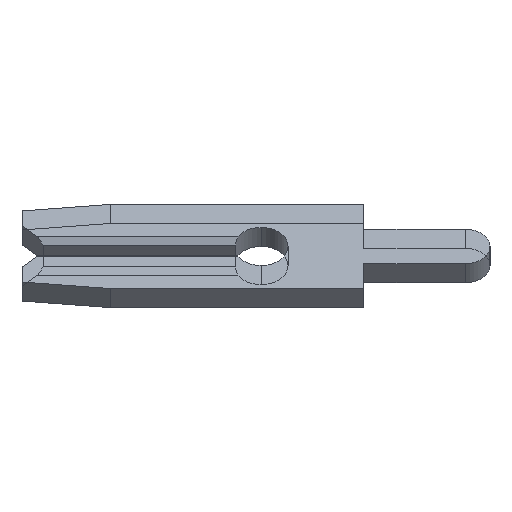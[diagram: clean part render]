
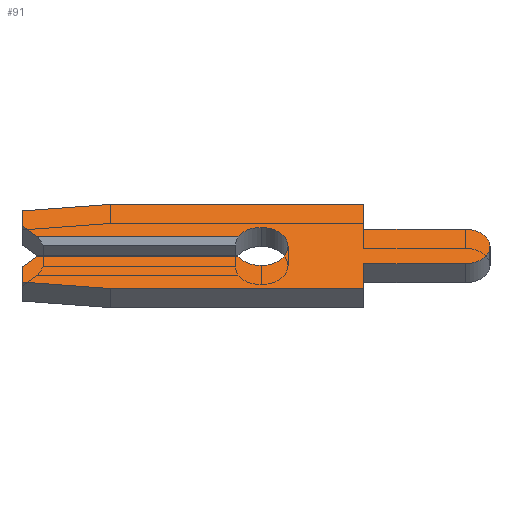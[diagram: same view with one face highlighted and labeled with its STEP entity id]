
A CAD part, left-side view. The second image highlights one B-rep face of the part: STEP entity #91.
In plain terms, the highlighted face is planar.
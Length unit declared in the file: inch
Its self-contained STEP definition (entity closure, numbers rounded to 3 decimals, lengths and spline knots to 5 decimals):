
#60 = CARTESIAN_POINT ( 'NONE',  ( -0.013, -0.099, -0.0235 ) ) ;
#91 = ADVANCED_FACE ( 'NONE', ( #1118 ), #2177, .F. ) ;
#99 = VERTEX_POINT ( 'NONE', #2155 ) ;
#103 = CARTESIAN_POINT ( 'NONE',  ( -0.013, 0.146, 0.0575 ) ) ;
#112 = CARTESIAN_POINT ( 'NONE',  ( -0.013, -0.099, 0.0235 ) ) ;
#117 = ORIENTED_EDGE ( 'NONE', *, *, #1726, .F. ) ;
#126 = VECTOR ( 'NONE', #705, 39.37008 ) ;
#244 = DIRECTION ( 'NONE',  ( -1., 0., 0. ) ) ;
#257 = CARTESIAN_POINT ( 'NONE',  ( -0.013, -0.099, -0.0575 ) ) ;
#270 = DIRECTION ( 'NONE',  ( 0., 0., -1. ) ) ;
#275 = ORIENTED_EDGE ( 'NONE', *, *, #1500, .F. ) ;
#277 = AXIS2_PLACEMENT_3D ( 'NONE', #1035, #1986, #2383 ) ;
#281 = VECTOR ( 'NONE', #2436, 39.37008 ) ;
#286 = VERTEX_POINT ( 'NONE', #1209 ) ;
#304 = CARTESIAN_POINT ( 'NONE',  ( -0.013, 0.231, 0.013 ) ) ;
#312 = VECTOR ( 'NONE', #2192, 39.37008 ) ;
#326 = EDGE_CURVE ( 'NONE', #1054, #760, #437, .T. ) ;
#342 = CIRCLE ( 'NONE', #898, 0.026 ) ;
#346 = CARTESIAN_POINT ( 'NONE',  ( -0.013, 0.216, -0.013 ) ) ;
#365 = LINE ( 'NONE', #1423, #1290 ) ;
#419 = LINE ( 'NONE', #2057, #1211 ) ;
#423 = DIRECTION ( 'NONE',  ( 0., 0., -1. ) ) ;
#432 = ORIENTED_EDGE ( 'NONE', *, *, #2236, .F. ) ;
#434 = VECTOR ( 'NONE', #1541, 39.37008 ) ;
#437 = LINE ( 'NONE', #1969, #2438 ) ;
#481 = EDGE_CURVE ( 'NONE', #649, #2296, #1342, .T. ) ;
#502 = LINE ( 'NONE', #1809, #1107 ) ;
#508 = CIRCLE ( 'NONE', #2370, 0.0235 ) ;
#511 = DIRECTION ( 'NONE',  ( -1., 0., 0. ) ) ;
#542 = LINE ( 'NONE', #908, #434 ) ;
#558 = ORIENTED_EDGE ( 'NONE', *, *, #858, .F. ) ;
#614 = DIRECTION ( 'NONE',  ( 0., -1., 0. ) ) ;
#634 = ORIENTED_EDGE ( 'NONE', *, *, #1562, .F. ) ;
#649 = VERTEX_POINT ( 'NONE', #60 ) ;
#651 = CARTESIAN_POINT ( 'NONE',  ( -0.013, 0., 0. ) ) ;
#661 = VECTOR ( 'NONE', #2313, 39.37008 ) ;
#692 = VERTEX_POINT ( 'NONE', #1614 ) ;
#705 = DIRECTION ( 'NONE',  ( 0., -1., 0. ) ) ;
#708 = CARTESIAN_POINT ( 'NONE',  ( -0.013, 0.02252, -0.013 ) ) ;
#726 = EDGE_CURVE ( 'NONE', #1320, #2247, #1497, .T. ) ;
#737 = CARTESIAN_POINT ( 'NONE',  ( -0.013, 0.231, -0.028 ) ) ;
#760 = VERTEX_POINT ( 'NONE', #2228 ) ;
#766 = CARTESIAN_POINT ( 'NONE',  ( -0.013, 0.2105, -0.0075 ) ) ;
#819 = LINE ( 'NONE', #766, #853 ) ;
#828 = EDGE_CURVE ( 'NONE', #692, #2247, #342, .T. ) ;
#845 = VERTEX_POINT ( 'NONE', #103 ) ;
#853 = VECTOR ( 'NONE', #1145, 39.37008 ) ;
#858 = EDGE_CURVE ( 'NONE', #1320, #1738, #1746, .T. ) ;
#898 = AXIS2_PLACEMENT_3D ( 'NONE', #2047, #511, #1663 ) ;
#908 = CARTESIAN_POINT ( 'NONE',  ( -0.013, 0., -0.013 ) ) ;
#970 = CARTESIAN_POINT ( 'NONE',  ( -0.013, 0.146, -0.0575 ) ) ;
#1035 = CARTESIAN_POINT ( 'NONE',  ( -0.013, 0., 0. ) ) ;
#1050 = CARTESIAN_POINT ( 'NONE',  ( -0.013, -0.1975, 0. ) ) ;
#1054 = VERTEX_POINT ( 'NONE', #112 ) ;
#1061 = VECTOR ( 'NONE', #1539, 39.37008 ) ;
#1098 = CARTESIAN_POINT ( 'NONE',  ( -0.013, 0.231, -0.04857 ) ) ;
#1106 = VECTOR ( 'NONE', #1156, 39.37008 ) ;
#1107 = VECTOR ( 'NONE', #1991, 39.37008 ) ;
#1118 = FACE_OUTER_BOUND ( 'NONE', #1835, .T. ) ;
#1127 = EDGE_CURVE ( 'NONE', #845, #99, #419, .T. ) ;
#1145 = DIRECTION ( 'NONE',  ( 0., -0.707, 0.707 ) ) ;
#1156 = DIRECTION ( 'NONE',  ( 0., 1., 0. ) ) ;
#1158 = ORIENTED_EDGE ( 'NONE', *, *, #1813, .F. ) ;
#1181 = DIRECTION ( 'NONE',  ( 0., 0., -1. ) ) ;
#1185 = CARTESIAN_POINT ( 'NONE',  ( -0.013, 0.231, 0.028 ) ) ;
#1202 = ORIENTED_EDGE ( 'NONE', *, *, #326, .F. ) ;
#1205 = VECTOR ( 'NONE', #2275, 39.37008 ) ;
#1206 = ORIENTED_EDGE ( 'NONE', *, *, #2458, .F. ) ;
#1209 = CARTESIAN_POINT ( 'NONE',  ( -0.013, 0., -0.026 ) ) ;
#1211 = VECTOR ( 'NONE', #1296, 39.37008 ) ;
#1233 = VERTEX_POINT ( 'NONE', #346 ) ;
#1245 = CARTESIAN_POINT ( 'NONE',  ( -0.013, 0.231, -0.028 ) ) ;
#1257 = CARTESIAN_POINT ( 'NONE',  ( -0.013, 0.231, 0.04857 ) ) ;
#1260 = ORIENTED_EDGE ( 'NONE', *, *, #828, .F. ) ;
#1290 = VECTOR ( 'NONE', #270, 39.37008 ) ;
#1296 = DIRECTION ( 'NONE',  ( 0., -1., 0. ) ) ;
#1320 = VERTEX_POINT ( 'NONE', #1929 ) ;
#1335 = EDGE_CURVE ( 'NONE', #2305, #2015, #1534, .T. ) ;
#1342 = LINE ( 'NONE', #257, #312 ) ;
#1367 = VERTEX_POINT ( 'NONE', #2285 ) ;
#1374 = CARTESIAN_POINT ( 'NONE',  ( -0.013, -0.099, -0.0235 ) ) ;
#1384 = DIRECTION ( 'NONE',  ( 0., 0., 1. ) ) ;
#1423 = CARTESIAN_POINT ( 'NONE',  ( -0.013, -0.099, 0.0575 ) ) ;
#1428 = EDGE_CURVE ( 'NONE', #2015, #1233, #819, .T. ) ;
#1436 = ORIENTED_EDGE ( 'NONE', *, *, #1127, .F. ) ;
#1442 = ORIENTED_EDGE ( 'NONE', *, *, #726, .T. ) ;
#1483 = CARTESIAN_POINT ( 'NONE',  ( -0.013, 0.2105, 0.0075 ) ) ;
#1497 = LINE ( 'NONE', #304, #126 ) ;
#1500 = EDGE_CURVE ( 'NONE', #2301, #286, #2125, .T. ) ;
#1528 = CIRCLE ( 'NONE', #2007, 0.026 ) ;
#1534 = LINE ( 'NONE', #737, #1205 ) ;
#1539 = DIRECTION ( 'NONE',  ( 0., 0., 1. ) ) ;
#1541 = DIRECTION ( 'NONE',  ( 0., -1., 0. ) ) ;
#1548 = CARTESIAN_POINT ( 'NONE',  ( -0.013, 0., 0. ) ) ;
#1562 = EDGE_CURVE ( 'NONE', #1738, #2212, #2016, .T. ) ;
#1570 = VECTOR ( 'NONE', #2343, 39.37008 ) ;
#1578 = CARTESIAN_POINT ( 'NONE',  ( -0.013, 0.146, -0.0575 ) ) ;
#1603 = DIRECTION ( 'NONE',  ( 1., 0., 0. ) ) ;
#1611 = VERTEX_POINT ( 'NONE', #1578 ) ;
#1614 = CARTESIAN_POINT ( 'NONE',  ( -0.013, 0., 0.026 ) ) ;
#1619 = ORIENTED_EDGE ( 'NONE', *, *, #1794, .F. ) ;
#1663 = DIRECTION ( 'NONE',  ( 0., 0., -1. ) ) ;
#1689 = LINE ( 'NONE', #2148, #1570 ) ;
#1692 = EDGE_CURVE ( 'NONE', #2212, #845, #1689, .T. ) ;
#1722 = AXIS2_PLACEMENT_3D ( 'NONE', #1548, #2128, #1181 ) ;
#1726 = EDGE_CURVE ( 'NONE', #2296, #1611, #2412, .T. ) ;
#1738 = VERTEX_POINT ( 'NONE', #1792 ) ;
#1746 = LINE ( 'NONE', #1483, #281 ) ;
#1792 = CARTESIAN_POINT ( 'NONE',  ( -0.013, 0.231, 0.028 ) ) ;
#1794 = EDGE_CURVE ( 'NONE', #286, #692, #1528, .T. ) ;
#1809 = CARTESIAN_POINT ( 'NONE',  ( -0.013, 0.231, -0.04857 ) ) ;
#1813 = EDGE_CURVE ( 'NONE', #760, #1367, #508, .T. ) ;
#1835 = EDGE_LOOP ( 'NONE', ( #1442, #1260, #1619, #275, #1206, #2242, #1996, #2179, #117, #2214, #2091, #1158, #1202, #432, #1436, #1898, #634, #558 ) ) ;
#1845 = LINE ( 'NONE', #1374, #1106 ) ;
#1869 = EDGE_CURVE ( 'NONE', #1611, #2305, #502, .T. ) ;
#1898 = ORIENTED_EDGE ( 'NONE', *, *, #1692, .F. ) ;
#1929 = CARTESIAN_POINT ( 'NONE',  ( -0.013, 0.216, 0.013 ) ) ;
#1969 = CARTESIAN_POINT ( 'NONE',  ( -0.013, -0.099, 0.0235 ) ) ;
#1986 = DIRECTION ( 'NONE',  ( 1., 0., 0. ) ) ;
#1991 = DIRECTION ( 'NONE',  ( 0., 0.995, 0.105 ) ) ;
#1996 = ORIENTED_EDGE ( 'NONE', *, *, #1335, .F. ) ;
#2007 = AXIS2_PLACEMENT_3D ( 'NONE', #651, #244, #423 ) ;
#2015 = VERTEX_POINT ( 'NONE', #1245 ) ;
#2016 = LINE ( 'NONE', #1185, #1061 ) ;
#2047 = CARTESIAN_POINT ( 'NONE',  ( -0.013, 0., 0. ) ) ;
#2057 = CARTESIAN_POINT ( 'NONE',  ( -0.013, 0.146, 0.0575 ) ) ;
#2091 = ORIENTED_EDGE ( 'NONE', *, *, #2445, .F. ) ;
#2125 = CIRCLE ( 'NONE', #1722, 0.026 ) ;
#2128 = DIRECTION ( 'NONE',  ( -1., 0., 0. ) ) ;
#2148 = CARTESIAN_POINT ( 'NONE',  ( -0.013, 0.231, 0.04857 ) ) ;
#2155 = CARTESIAN_POINT ( 'NONE',  ( -0.013, -0.099, 0.0575 ) ) ;
#2177 = PLANE ( 'NONE',  #277 ) ;
#2179 = ORIENTED_EDGE ( 'NONE', *, *, #1869, .F. ) ;
#2192 = DIRECTION ( 'NONE',  ( 0., 0., -1. ) ) ;
#2212 = VERTEX_POINT ( 'NONE', #1257 ) ;
#2214 = ORIENTED_EDGE ( 'NONE', *, *, #481, .F. ) ;
#2228 = CARTESIAN_POINT ( 'NONE',  ( -0.013, -0.1975, 0.0235 ) ) ;
#2236 = EDGE_CURVE ( 'NONE', #99, #1054, #365, .T. ) ;
#2242 = ORIENTED_EDGE ( 'NONE', *, *, #1428, .F. ) ;
#2247 = VERTEX_POINT ( 'NONE', #2433 ) ;
#2275 = DIRECTION ( 'NONE',  ( 0., 0., 1. ) ) ;
#2285 = CARTESIAN_POINT ( 'NONE',  ( -0.013, -0.1975, -0.0235 ) ) ;
#2296 = VERTEX_POINT ( 'NONE', #2424 ) ;
#2301 = VERTEX_POINT ( 'NONE', #708 ) ;
#2305 = VERTEX_POINT ( 'NONE', #1098 ) ;
#2313 = DIRECTION ( 'NONE',  ( 0., 1., 0. ) ) ;
#2343 = DIRECTION ( 'NONE',  ( 0., -0.995, 0.105 ) ) ;
#2370 = AXIS2_PLACEMENT_3D ( 'NONE', #1050, #1603, #1384 ) ;
#2383 = DIRECTION ( 'NONE',  ( 0., 0., -1. ) ) ;
#2412 = LINE ( 'NONE', #970, #661 ) ;
#2424 = CARTESIAN_POINT ( 'NONE',  ( -0.013, -0.099, -0.0575 ) ) ;
#2433 = CARTESIAN_POINT ( 'NONE',  ( -0.013, 0.02252, 0.013 ) ) ;
#2436 = DIRECTION ( 'NONE',  ( 0., 0.707, 0.707 ) ) ;
#2438 = VECTOR ( 'NONE', #614, 39.37008 ) ;
#2445 = EDGE_CURVE ( 'NONE', #1367, #649, #1845, .T. ) ;
#2458 = EDGE_CURVE ( 'NONE', #1233, #2301, #542, .T. ) ;
